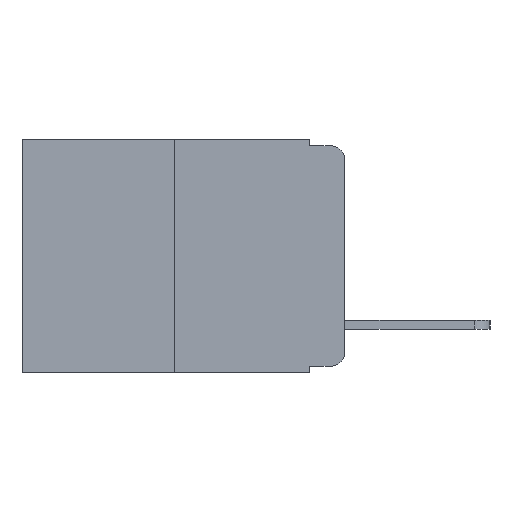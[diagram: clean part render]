
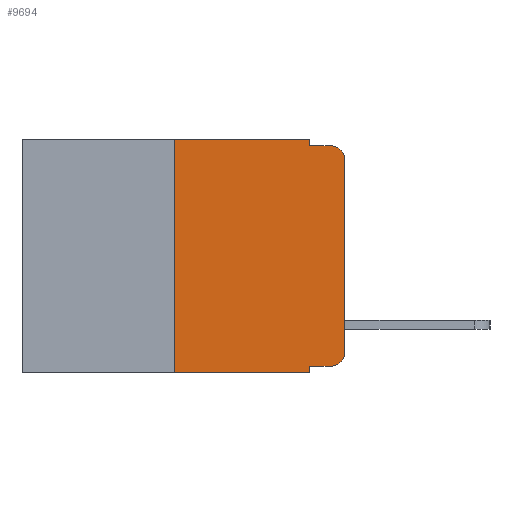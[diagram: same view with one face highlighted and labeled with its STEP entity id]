
A CAD part, left-side view. The second image highlights one B-rep face of the part: STEP entity #9694.
In plain terms, the highlighted planar face has unit normal (-1, 0, 0).
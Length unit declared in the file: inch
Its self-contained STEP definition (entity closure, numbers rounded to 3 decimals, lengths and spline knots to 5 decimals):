
#4 = LINE ( 'NONE', #9013, #5645 ) ;
#8 = ORIENTED_EDGE ( 'NONE', *, *, #2497, .T. ) ;
#133 = ORIENTED_EDGE ( 'NONE', *, *, #2518, .F. ) ;
#156 = CARTESIAN_POINT ( 'NONE',  ( 0., 0., 0. ) ) ;
#196 = VECTOR ( 'NONE', #1993, 39.37008 ) ;
#218 = ORIENTED_EDGE ( 'NONE', *, *, #2555, .F. ) ;
#233 = DIRECTION ( 'NONE',  ( 0., 0., -1. ) ) ;
#244 = ORIENTED_EDGE ( 'NONE', *, *, #6381, .F. ) ;
#362 = ORIENTED_EDGE ( 'NONE', *, *, #2561, .F. ) ;
#364 = VERTEX_POINT ( 'NONE', #4260 ) ;
#388 = ORIENTED_EDGE ( 'NONE', *, *, #9452, .T. ) ;
#407 = ORIENTED_EDGE ( 'NONE', *, *, #2572, .F. ) ;
#588 = VERTEX_POINT ( 'NONE', #5188 ) ;
#617 = ORIENTED_EDGE ( 'NONE', *, *, #2575, .T. ) ;
#658 = FACE_OUTER_BOUND ( 'NONE', #2351, .T. ) ;
#873 = ORIENTED_EDGE ( 'NONE', *, *, #2577, .T. ) ;
#991 = DIRECTION ( 'NONE',  ( 0., -1., 0. ) ) ;
#1202 = CARTESIAN_POINT ( 'NONE',  ( 0., 0.051, 0. ) ) ;
#1618 = LINE ( 'NONE', #12825, #7739 ) ;
#1894 = AXIS2_PLACEMENT_3D ( 'NONE', #4998, #4890, #3917 ) ;
#1918 = AXIS2_PLACEMENT_3D ( 'NONE', #3301, #3044, #3337 ) ;
#1985 = VECTOR ( 'NONE', #233, 39.37008 ) ;
#1993 = DIRECTION ( 'NONE',  ( 0., 0., 1. ) ) ;
#2116 = VERTEX_POINT ( 'NONE', #5545 ) ;
#2337 = CARTESIAN_POINT ( 'NONE',  ( 0., 0., -0.03 ) ) ;
#2351 = EDGE_LOOP ( 'NONE', ( #7515, #8, #133, #218, #244, #362, #388, #407, #617, #873 ) ) ;
#2353 = DIRECTION ( 'NONE',  ( 0., -1., 0. ) ) ;
#2490 = EDGE_CURVE ( 'NONE', #6888, #8256, #11947, .T. ) ;
#2497 = EDGE_CURVE ( 'NONE', #8256, #10500, #9451, .T. ) ;
#2518 = EDGE_CURVE ( 'NONE', #4126, #10500, #3094, .T. ) ;
#2555 = EDGE_CURVE ( 'NONE', #3022, #4126, #13224, .T. ) ;
#2561 = EDGE_CURVE ( 'NONE', #2116, #364, #12952, .T. ) ;
#2572 = EDGE_CURVE ( 'NONE', #588, #7809, #12665, .T. ) ;
#2575 = EDGE_CURVE ( 'NONE', #588, #11800, #1618, .T. ) ;
#2577 = EDGE_CURVE ( 'NONE', #11800, #6888, #7352, .T. ) ;
#3022 = VERTEX_POINT ( 'NONE', #1202 ) ;
#3044 = DIRECTION ( 'NONE',  ( -1., 0., 0. ) ) ;
#3094 = LINE ( 'NONE', #3792, #6140 ) ;
#3301 = CARTESIAN_POINT ( 'NONE',  ( 0., 0.02, -0.03 ) ) ;
#3337 = DIRECTION ( 'NONE',  ( 0., 0., -1. ) ) ;
#3792 = CARTESIAN_POINT ( 'NONE',  ( 0., 0.051, -0.01 ) ) ;
#3917 = DIRECTION ( 'NONE',  ( 0., 0., -1. ) ) ;
#4126 = VERTEX_POINT ( 'NONE', #11128 ) ;
#4260 = CARTESIAN_POINT ( 'NONE',  ( 0., 0.25, 0. ) ) ;
#4336 = DIRECTION ( 'NONE',  ( 1., 0., 0. ) ) ;
#4355 = DIRECTION ( 'NONE',  ( 0., -1., 0. ) ) ;
#4668 = DIRECTION ( 'NONE',  ( 0., 0., -1. ) ) ;
#4751 = CARTESIAN_POINT ( 'NONE',  ( 0., 0.02, -0.333 ) ) ;
#4758 = VECTOR ( 'NONE', #12076, 39.37008 ) ;
#4890 = DIRECTION ( 'NONE',  ( -1., 0., 0. ) ) ;
#4998 = CARTESIAN_POINT ( 'NONE',  ( 0., 0.02, -0.313 ) ) ;
#5188 = CARTESIAN_POINT ( 'NONE',  ( 0., 0.051, -0.333 ) ) ;
#5545 = CARTESIAN_POINT ( 'NONE',  ( 0., 0.25, -0.343 ) ) ;
#5627 = AXIS2_PLACEMENT_3D ( 'NONE', #13416, #4336, #4668 ) ;
#5645 = VECTOR ( 'NONE', #4355, 39.37008 ) ;
#5989 = LINE ( 'NONE', #6213, #11836 ) ;
#6140 = VECTOR ( 'NONE', #2353, 39.37008 ) ;
#6213 = CARTESIAN_POINT ( 'NONE',  ( 0., 0.473, -0.343 ) ) ;
#6270 = CARTESIAN_POINT ( 'NONE',  ( 0., 0.051, 0. ) ) ;
#6381 = EDGE_CURVE ( 'NONE', #364, #3022, #4, .T. ) ;
#6888 = VERTEX_POINT ( 'NONE', #8307 ) ;
#7352 = CIRCLE ( 'NONE', #1894, 0.02 ) ;
#7515 = ORIENTED_EDGE ( 'NONE', *, *, #2490, .T. ) ;
#7739 = VECTOR ( 'NONE', #11978, 39.37008 ) ;
#7809 = VERTEX_POINT ( 'NONE', #12666 ) ;
#8256 = VERTEX_POINT ( 'NONE', #2337 ) ;
#8307 = CARTESIAN_POINT ( 'NONE',  ( 0., 0., -0.313 ) ) ;
#9013 = CARTESIAN_POINT ( 'NONE',  ( 0., 0.473, 0. ) ) ;
#9451 = CIRCLE ( 'NONE', #1918, 0.02 ) ;
#9452 = EDGE_CURVE ( 'NONE', #2116, #7809, #5989, .T. ) ;
#9694 = ADVANCED_FACE ( 'NONE', ( #658 ), #12294, .F. ) ;
#10302 = VECTOR ( 'NONE', #12551, 39.37008 ) ;
#10500 = VERTEX_POINT ( 'NONE', #12945 ) ;
#11128 = CARTESIAN_POINT ( 'NONE',  ( 0., 0.051, -0.01 ) ) ;
#11417 = CARTESIAN_POINT ( 'NONE',  ( 0., 0.051, 0. ) ) ;
#11800 = VERTEX_POINT ( 'NONE', #4751 ) ;
#11836 = VECTOR ( 'NONE', #991, 39.37008 ) ;
#11917 = CARTESIAN_POINT ( 'NONE',  ( 0., 0.25, 0. ) ) ;
#11947 = LINE ( 'NONE', #156, #196 ) ;
#11978 = DIRECTION ( 'NONE',  ( 0., -1., 0. ) ) ;
#12076 = DIRECTION ( 'NONE',  ( 0., 0., 1. ) ) ;
#12294 = PLANE ( 'NONE',  #5627 ) ;
#12551 = DIRECTION ( 'NONE',  ( 0., 0., -1. ) ) ;
#12665 = LINE ( 'NONE', #6270, #10302 ) ;
#12666 = CARTESIAN_POINT ( 'NONE',  ( 0., 0.051, -0.343 ) ) ;
#12825 = CARTESIAN_POINT ( 'NONE',  ( 0., 0.051, -0.333 ) ) ;
#12945 = CARTESIAN_POINT ( 'NONE',  ( 0., 0.02, -0.01 ) ) ;
#12952 = LINE ( 'NONE', #11917, #4758 ) ;
#13224 = LINE ( 'NONE', #11417, #1985 ) ;
#13416 = CARTESIAN_POINT ( 'NONE',  ( 0., 0.473, 0. ) ) ;
